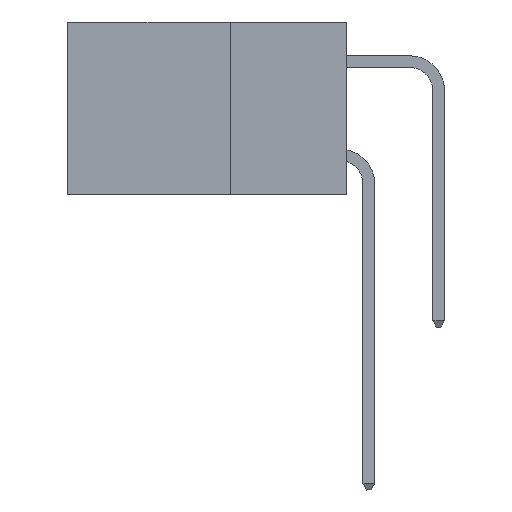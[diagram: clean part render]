
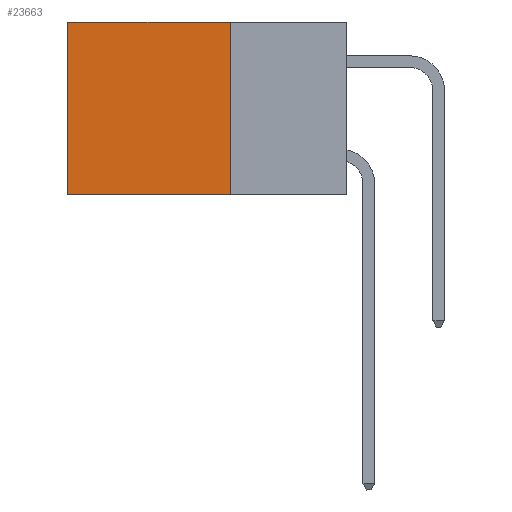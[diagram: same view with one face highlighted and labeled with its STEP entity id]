
A CAD part, left-side view. The second image highlights one B-rep face of the part: STEP entity #23663.
In plain terms, the highlighted planar face has unit normal (-1, 0, 0).
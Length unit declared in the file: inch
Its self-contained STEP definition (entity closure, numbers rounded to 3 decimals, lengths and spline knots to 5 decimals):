
#901 = LINE ( 'NONE', #12369, #19958 ) ;
#1038 = ORIENTED_EDGE ( 'NONE', *, *, #13818, .F. ) ;
#1728 = ORIENTED_EDGE ( 'NONE', *, *, #23248, .T. ) ;
#1800 = VERTEX_POINT ( 'NONE', #15445 ) ;
#4675 = VERTEX_POINT ( 'NONE', #19598 ) ;
#4737 = DIRECTION ( 'NONE',  ( 0., 1., 0. ) ) ;
#4841 = CARTESIAN_POINT ( 'NONE',  ( 0.2875, 0.25, 0. ) ) ;
#5024 = EDGE_LOOP ( 'NONE', ( #1728, #13669, #1038, #14723 ) ) ;
#5501 = PLANE ( 'NONE',  #7782 ) ;
#7438 = DIRECTION ( 'NONE',  ( 0., 0., -1. ) ) ;
#7500 = LINE ( 'NONE', #12796, #16417 ) ;
#7782 = AXIS2_PLACEMENT_3D ( 'NONE', #16901, #18815, #7438 ) ;
#8160 = VECTOR ( 'NONE', #17616, 39.37008 ) ;
#8371 = VERTEX_POINT ( 'NONE', #19514 ) ;
#8698 = EDGE_CURVE ( 'NONE', #20826, #8371, #7500, .T. ) ;
#8965 = DIRECTION ( 'NONE',  ( 0., 1., 0. ) ) ;
#11383 = VECTOR ( 'NONE', #15600, 39.37008 ) ;
#12369 = CARTESIAN_POINT ( 'NONE',  ( 0.2875, 0.25, -0.37 ) ) ;
#12796 = CARTESIAN_POINT ( 'NONE',  ( 0.2875, 0.25, 0. ) ) ;
#13669 = ORIENTED_EDGE ( 'NONE', *, *, #14037, .F. ) ;
#13699 = CARTESIAN_POINT ( 'NONE',  ( 0.2875, 0.25, 0. ) ) ;
#13809 = FACE_OUTER_BOUND ( 'NONE', #5024, .T. ) ;
#13818 = EDGE_CURVE ( 'NONE', #20826, #4675, #20851, .T. ) ;
#14037 = EDGE_CURVE ( 'NONE', #4675, #1800, #901, .T. ) ;
#14723 = ORIENTED_EDGE ( 'NONE', *, *, #8698, .T. ) ;
#15445 = CARTESIAN_POINT ( 'NONE',  ( 0.2875, 0.6, -0.37 ) ) ;
#15600 = DIRECTION ( 'NONE',  ( 0., 0., -1. ) ) ;
#16417 = VECTOR ( 'NONE', #8965, 39.37008 ) ;
#16901 = CARTESIAN_POINT ( 'NONE',  ( 0.2875, 0.25, 0. ) ) ;
#17616 = DIRECTION ( 'NONE',  ( 0., 0., -1. ) ) ;
#17685 = LINE ( 'NONE', #23239, #8160 ) ;
#18815 = DIRECTION ( 'NONE',  ( 1., 0., 0. ) ) ;
#19514 = CARTESIAN_POINT ( 'NONE',  ( 0.2875, 0.6, 0. ) ) ;
#19598 = CARTESIAN_POINT ( 'NONE',  ( 0.2875, 0.25, -0.37 ) ) ;
#19958 = VECTOR ( 'NONE', #4737, 39.37008 ) ;
#20826 = VERTEX_POINT ( 'NONE', #4841 ) ;
#20851 = LINE ( 'NONE', #13699, #11383 ) ;
#23239 = CARTESIAN_POINT ( 'NONE',  ( 0.2875, 0.6, 0. ) ) ;
#23248 = EDGE_CURVE ( 'NONE', #8371, #1800, #17685, .T. ) ;
#23663 = ADVANCED_FACE ( 'NONE', ( #13809 ), #5501, .F. ) ;
